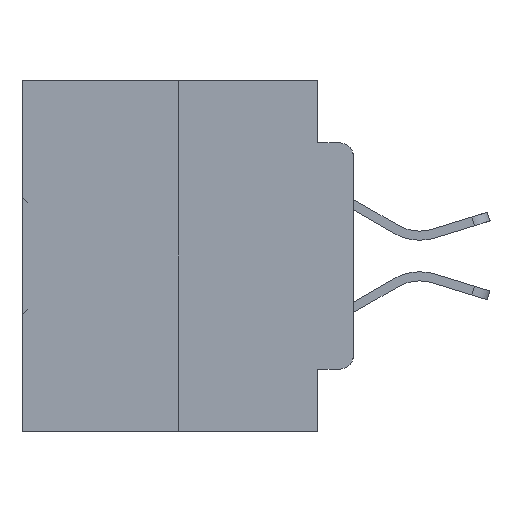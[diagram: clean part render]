
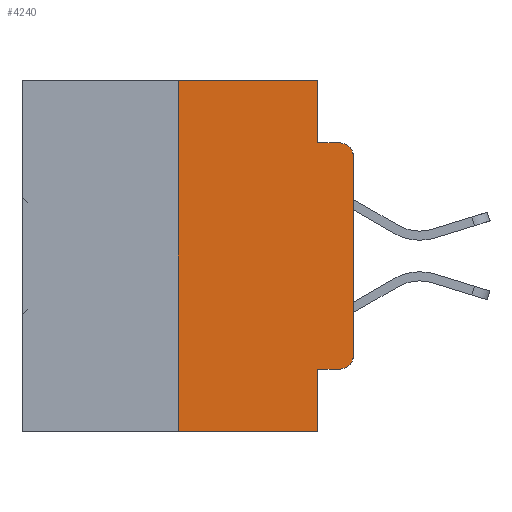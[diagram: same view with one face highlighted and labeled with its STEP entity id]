
A CAD part, left-side view. The second image highlights one B-rep face of the part: STEP entity #4240.
In plain terms, the highlighted planar face has unit normal (-1, 0, 0).
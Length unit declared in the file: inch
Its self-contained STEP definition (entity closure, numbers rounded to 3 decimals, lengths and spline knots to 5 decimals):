
#978 = ORIENTED_EDGE ( 'NONE', *, *, #16875, .T. ) ;
#999 = CARTESIAN_POINT ( 'NONE',  ( 0., 0.02, -0.3915 ) ) ;
#1475 = VERTEX_POINT ( 'NONE', #10394 ) ;
#1826 = EDGE_CURVE ( 'NONE', #35428, #25365, #16868, .T. ) ;
#2483 = AXIS2_PLACEMENT_3D ( 'NONE', #999, #20667, #3855 ) ;
#2724 = VECTOR ( 'NONE', #23185, 39.37008 ) ;
#3211 = ORIENTED_EDGE ( 'NONE', *, *, #18965, .T. ) ;
#3373 = CARTESIAN_POINT ( 'NONE',  ( 0., 0.051, -0.4115 ) ) ;
#3710 = EDGE_CURVE ( 'NONE', #27792, #25365, #23321, .T. ) ;
#3855 = DIRECTION ( 'NONE',  ( 0., 0., -1. ) ) ;
#4107 = LINE ( 'NONE', #13658, #33061 ) ;
#4240 = ADVANCED_FACE ( 'NONE', ( #35550 ), #7771, .F. ) ;
#4835 = VERTEX_POINT ( 'NONE', #24872 ) ;
#5009 = ORIENTED_EDGE ( 'NONE', *, *, #15198, .T. ) ;
#5572 = DIRECTION ( 'NONE',  ( 1., 0., 0. ) ) ;
#6009 = VERTEX_POINT ( 'NONE', #35843 ) ;
#6843 = EDGE_CURVE ( 'NONE', #6009, #20235, #25149, .T. ) ;
#6960 = VECTOR ( 'NONE', #16393, 39.37008 ) ;
#7183 = ORIENTED_EDGE ( 'NONE', *, *, #22615, .F. ) ;
#7382 = CARTESIAN_POINT ( 'NONE',  ( 0., 0.25, 0. ) ) ;
#7641 = CARTESIAN_POINT ( 'NONE',  ( 0., 0.25, 0. ) ) ;
#7771 = PLANE ( 'NONE',  #24580 ) ;
#8736 = VERTEX_POINT ( 'NONE', #7641 ) ;
#9025 = AXIS2_PLACEMENT_3D ( 'NONE', #33436, #16643, #36223 ) ;
#9057 = CARTESIAN_POINT ( 'NONE',  ( 0., 0.473, -0.5 ) ) ;
#9342 = ORIENTED_EDGE ( 'NONE', *, *, #3710, .T. ) ;
#9810 = ORIENTED_EDGE ( 'NONE', *, *, #23228, .F. ) ;
#10394 = CARTESIAN_POINT ( 'NONE',  ( 0., 0., -0.3915 ) ) ;
#10601 = DIRECTION ( 'NONE',  ( 0., 0., 1. ) ) ;
#10849 = LINE ( 'NONE', #24325, #16569 ) ;
#12157 = CARTESIAN_POINT ( 'NONE',  ( 0., 0.051, -0.0885 ) ) ;
#13244 = VECTOR ( 'NONE', #14013, 39.37008 ) ;
#13505 = CARTESIAN_POINT ( 'NONE',  ( 0., 0.051, 0. ) ) ;
#13658 = CARTESIAN_POINT ( 'NONE',  ( 0., 0.051, -0.4115 ) ) ;
#14013 = DIRECTION ( 'NONE',  ( 0., 0., -1. ) ) ;
#14396 = LINE ( 'NONE', #27547, #6960 ) ;
#15009 = LINE ( 'NONE', #28024, #13244 ) ;
#15198 = EDGE_CURVE ( 'NONE', #4835, #1475, #29522, .T. ) ;
#15793 = LINE ( 'NONE', #7382, #35581 ) ;
#16002 = VECTOR ( 'NONE', #23011, 39.37008 ) ;
#16365 = CARTESIAN_POINT ( 'NONE',  ( 0., 0., -0.1085 ) ) ;
#16393 = DIRECTION ( 'NONE',  ( 0., -1., 0. ) ) ;
#16569 = VECTOR ( 'NONE', #32776, 39.37008 ) ;
#16643 = DIRECTION ( 'NONE',  ( -1., 0., 0. ) ) ;
#16868 = LINE ( 'NONE', #20197, #16002 ) ;
#16875 = EDGE_CURVE ( 'NONE', #1475, #27792, #20599, .T. ) ;
#17620 = VERTEX_POINT ( 'NONE', #13505 ) ;
#18543 = DIRECTION ( 'NONE',  ( 0., 0., 1. ) ) ;
#18965 = EDGE_CURVE ( 'NONE', #21453, #4835, #4107, .T. ) ;
#19463 = ORIENTED_EDGE ( 'NONE', *, *, #1826, .F. ) ;
#19715 = VECTOR ( 'NONE', #10601, 39.37008 ) ;
#20197 = CARTESIAN_POINT ( 'NONE',  ( 0., 0.051, -0.0885 ) ) ;
#20235 = VERTEX_POINT ( 'NONE', #31317 ) ;
#20599 = LINE ( 'NONE', #21792, #19715 ) ;
#20667 = DIRECTION ( 'NONE',  ( -1., 0., 0. ) ) ;
#21453 = VERTEX_POINT ( 'NONE', #3373 ) ;
#21792 = CARTESIAN_POINT ( 'NONE',  ( 0., 0., 0. ) ) ;
#22615 = EDGE_CURVE ( 'NONE', #8736, #17620, #14396, .T. ) ;
#23011 = DIRECTION ( 'NONE',  ( 0., -1., 0. ) ) ;
#23185 = DIRECTION ( 'NONE',  ( 0., -1., 0. ) ) ;
#23228 = EDGE_CURVE ( 'NONE', #21453, #20235, #10849, .T. ) ;
#23321 = CIRCLE ( 'NONE', #9025, 0.02 ) ;
#23879 = ORIENTED_EDGE ( 'NONE', *, *, #6843, .T. ) ;
#24325 = CARTESIAN_POINT ( 'NONE',  ( 0., 0.051, 0. ) ) ;
#24580 = AXIS2_PLACEMENT_3D ( 'NONE', #33033, #5572, #25207 ) ;
#24872 = CARTESIAN_POINT ( 'NONE',  ( 0., 0.02, -0.4115 ) ) ;
#25149 = LINE ( 'NONE', #9057, #2724 ) ;
#25207 = DIRECTION ( 'NONE',  ( 0., 0., -1. ) ) ;
#25365 = VERTEX_POINT ( 'NONE', #30920 ) ;
#27547 = CARTESIAN_POINT ( 'NONE',  ( 0., 0.473, 0. ) ) ;
#27792 = VERTEX_POINT ( 'NONE', #16365 ) ;
#27805 = ORIENTED_EDGE ( 'NONE', *, *, #32627, .F. ) ;
#28024 = CARTESIAN_POINT ( 'NONE',  ( 0., 0.051, 0. ) ) ;
#28862 = EDGE_CURVE ( 'NONE', #6009, #8736, #15793, .T. ) ;
#29522 = CIRCLE ( 'NONE', #2483, 0.02 ) ;
#29581 = ORIENTED_EDGE ( 'NONE', *, *, #28862, .F. ) ;
#30920 = CARTESIAN_POINT ( 'NONE',  ( 0., 0.02, -0.0885 ) ) ;
#31317 = CARTESIAN_POINT ( 'NONE',  ( 0., 0.051, -0.5 ) ) ;
#32627 = EDGE_CURVE ( 'NONE', #17620, #35428, #15009, .T. ) ;
#32776 = DIRECTION ( 'NONE',  ( 0., 0., -1. ) ) ;
#32812 = EDGE_LOOP ( 'NONE', ( #978, #9342, #19463, #27805, #7183, #29581, #23879, #9810, #3211, #5009 ) ) ;
#33033 = CARTESIAN_POINT ( 'NONE',  ( 0., 0.473, 0. ) ) ;
#33061 = VECTOR ( 'NONE', #36090, 39.37008 ) ;
#33436 = CARTESIAN_POINT ( 'NONE',  ( 0., 0.02, -0.1085 ) ) ;
#35428 = VERTEX_POINT ( 'NONE', #12157 ) ;
#35550 = FACE_OUTER_BOUND ( 'NONE', #32812, .T. ) ;
#35581 = VECTOR ( 'NONE', #18543, 39.37008 ) ;
#35843 = CARTESIAN_POINT ( 'NONE',  ( 0., 0.25, -0.5 ) ) ;
#36090 = DIRECTION ( 'NONE',  ( 0., -1., 0. ) ) ;
#36223 = DIRECTION ( 'NONE',  ( 0., 0., -1. ) ) ;
